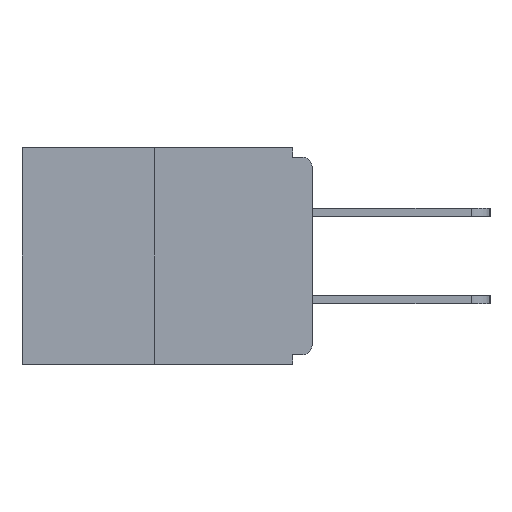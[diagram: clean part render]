
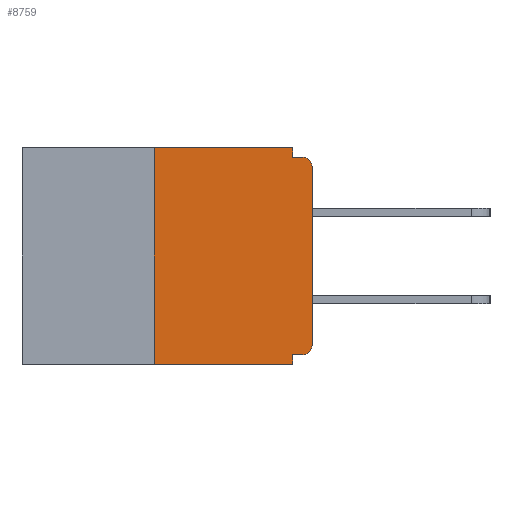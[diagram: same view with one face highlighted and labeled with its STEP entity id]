
A CAD part, left-side view. The second image highlights one B-rep face of the part: STEP entity #8759.
In plain terms, the highlighted planar face has unit normal (-1, 0, 0).
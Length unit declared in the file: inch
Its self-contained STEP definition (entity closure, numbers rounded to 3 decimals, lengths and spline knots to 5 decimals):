
#28 = ORIENTED_EDGE ( 'NONE', *, *, #10437, .F. ) ;
#290 = DIRECTION ( 'NONE',  ( 0., -1., 0. ) ) ;
#306 = LINE ( 'NONE', #11990, #9862 ) ;
#543 = DIRECTION ( 'NONE',  ( 0., 0., -1. ) ) ;
#648 = VERTEX_POINT ( 'NONE', #5772 ) ;
#1093 = VERTEX_POINT ( 'NONE', #7994 ) ;
#1629 = LINE ( 'NONE', #5684, #9766 ) ;
#1673 = AXIS2_PLACEMENT_3D ( 'NONE', #9040, #13165, #12157 ) ;
#1698 = DIRECTION ( 'NONE',  ( 0., 0., -1. ) ) ;
#1803 = CARTESIAN_POINT ( 'NONE',  ( 0., 0.031, -0.328 ) ) ;
#2079 = CARTESIAN_POINT ( 'NONE',  ( 0., 0.015, -0.328 ) ) ;
#2335 = ORIENTED_EDGE ( 'NONE', *, *, #8052, .T. ) ;
#2463 = ORIENTED_EDGE ( 'NONE', *, *, #7487, .F. ) ;
#2608 = VERTEX_POINT ( 'NONE', #1803 ) ;
#2695 = DIRECTION ( 'NONE',  ( 0., 0., -1. ) ) ;
#2817 = EDGE_CURVE ( 'NONE', #6323, #648, #8437, .T. ) ;
#3009 = EDGE_CURVE ( 'NONE', #8001, #4327, #10354, .T. ) ;
#3018 = DIRECTION ( 'NONE',  ( 0., 0., 1. ) ) ;
#3158 = VECTOR ( 'NONE', #290, 39.37008 ) ;
#3190 = CARTESIAN_POINT ( 'NONE',  ( 0., 0., -0.015 ) ) ;
#3207 = EDGE_CURVE ( 'NONE', #4444, #6323, #4548, .T. ) ;
#3313 = VECTOR ( 'NONE', #8909, 39.37008 ) ;
#3400 = CARTESIAN_POINT ( 'NONE',  ( 0., 0.25, -0.343 ) ) ;
#3809 = DIRECTION ( 'NONE',  ( -1., 0., 0. ) ) ;
#4262 = CARTESIAN_POINT ( 'NONE',  ( 0., 0.46, -0.343 ) ) ;
#4326 = ORIENTED_EDGE ( 'NONE', *, *, #5638, .T. ) ;
#4327 = VERTEX_POINT ( 'NONE', #8380 ) ;
#4334 = CARTESIAN_POINT ( 'NONE',  ( 0., 0.015, -0.313 ) ) ;
#4444 = VERTEX_POINT ( 'NONE', #11571 ) ;
#4548 = LINE ( 'NONE', #12788, #5196 ) ;
#4572 = EDGE_CURVE ( 'NONE', #6795, #1093, #4666, .T. ) ;
#4666 = CIRCLE ( 'NONE', #9776, 0.015 ) ;
#4780 = CARTESIAN_POINT ( 'NONE',  ( 0., 0.031, 0. ) ) ;
#5086 = EDGE_CURVE ( 'NONE', #6795, #2608, #6924, .T. ) ;
#5196 = VECTOR ( 'NONE', #8714, 39.37008 ) ;
#5532 = ORIENTED_EDGE ( 'NONE', *, *, #2817, .F. ) ;
#5638 = EDGE_CURVE ( 'NONE', #1093, #9898, #7403, .T. ) ;
#5684 = CARTESIAN_POINT ( 'NONE',  ( 0., 0.031, -0.343 ) ) ;
#5772 = CARTESIAN_POINT ( 'NONE',  ( 0., 0.031, -0.015 ) ) ;
#5785 = VERTEX_POINT ( 'NONE', #6125 ) ;
#5816 = AXIS2_PLACEMENT_3D ( 'NONE', #6819, #3809, #1698 ) ;
#5965 = ORIENTED_EDGE ( 'NONE', *, *, #3009, .T. ) ;
#5969 = DIRECTION ( 'NONE',  ( 0., 0., 1. ) ) ;
#5979 = ORIENTED_EDGE ( 'NONE', *, *, #3207, .F. ) ;
#6125 = CARTESIAN_POINT ( 'NONE',  ( 0., 0.015, -0.015 ) ) ;
#6323 = VERTEX_POINT ( 'NONE', #9615 ) ;
#6329 = CARTESIAN_POINT ( 'NONE',  ( 0., 0., -0.328 ) ) ;
#6428 = ORIENTED_EDGE ( 'NONE', *, *, #5086, .F. ) ;
#6795 = VERTEX_POINT ( 'NONE', #2079 ) ;
#6819 = CARTESIAN_POINT ( 'NONE',  ( 0., 0.015, -0.03 ) ) ;
#6924 = LINE ( 'NONE', #6329, #7083 ) ;
#7083 = VECTOR ( 'NONE', #7292, 39.37008 ) ;
#7292 = DIRECTION ( 'NONE',  ( 0., 1., 0. ) ) ;
#7403 = LINE ( 'NONE', #13097, #9644 ) ;
#7487 = EDGE_CURVE ( 'NONE', #2608, #4327, #1629, .T. ) ;
#7907 = EDGE_LOOP ( 'NONE', ( #5979, #10758, #5965, #2463, #6428, #11333, #4326, #2335, #28, #5532 ) ) ;
#7994 = CARTESIAN_POINT ( 'NONE',  ( 0., 0., -0.313 ) ) ;
#8001 = VERTEX_POINT ( 'NONE', #3400 ) ;
#8052 = EDGE_CURVE ( 'NONE', #9898, #5785, #12489, .T. ) ;
#8104 = VECTOR ( 'NONE', #11373, 39.37008 ) ;
#8279 = LINE ( 'NONE', #3190, #8104 ) ;
#8380 = CARTESIAN_POINT ( 'NONE',  ( 0., 0.031, -0.343 ) ) ;
#8437 = LINE ( 'NONE', #4780, #3313 ) ;
#8714 = DIRECTION ( 'NONE',  ( 0., -1., 0. ) ) ;
#8759 = ADVANCED_FACE ( 'NONE', ( #9438 ), #11027, .F. ) ;
#8909 = DIRECTION ( 'NONE',  ( 0., 0., -1. ) ) ;
#9040 = CARTESIAN_POINT ( 'NONE',  ( 0., 0.46, 0. ) ) ;
#9438 = FACE_OUTER_BOUND ( 'NONE', #7907, .T. ) ;
#9615 = CARTESIAN_POINT ( 'NONE',  ( 0., 0.031, 0. ) ) ;
#9643 = EDGE_CURVE ( 'NONE', #8001, #4444, #306, .T. ) ;
#9644 = VECTOR ( 'NONE', #3018, 39.37008 ) ;
#9766 = VECTOR ( 'NONE', #2695, 39.37008 ) ;
#9776 = AXIS2_PLACEMENT_3D ( 'NONE', #4334, #12557, #543 ) ;
#9862 = VECTOR ( 'NONE', #5969, 39.37008 ) ;
#9898 = VERTEX_POINT ( 'NONE', #11080 ) ;
#10354 = LINE ( 'NONE', #4262, #3158 ) ;
#10437 = EDGE_CURVE ( 'NONE', #648, #5785, #8279, .T. ) ;
#10758 = ORIENTED_EDGE ( 'NONE', *, *, #9643, .F. ) ;
#11027 = PLANE ( 'NONE',  #1673 ) ;
#11080 = CARTESIAN_POINT ( 'NONE',  ( 0., 0., -0.03 ) ) ;
#11333 = ORIENTED_EDGE ( 'NONE', *, *, #4572, .T. ) ;
#11373 = DIRECTION ( 'NONE',  ( 0., -1., 0. ) ) ;
#11571 = CARTESIAN_POINT ( 'NONE',  ( 0., 0.25, 0. ) ) ;
#11990 = CARTESIAN_POINT ( 'NONE',  ( 0., 0.25, 0. ) ) ;
#12157 = DIRECTION ( 'NONE',  ( 0., 0., -1. ) ) ;
#12489 = CIRCLE ( 'NONE', #5816, 0.015 ) ;
#12557 = DIRECTION ( 'NONE',  ( -1., 0., 0. ) ) ;
#12788 = CARTESIAN_POINT ( 'NONE',  ( 0., 0.46, 0. ) ) ;
#13097 = CARTESIAN_POINT ( 'NONE',  ( 0., 0., 0. ) ) ;
#13165 = DIRECTION ( 'NONE',  ( 1., 0., 0. ) ) ;
